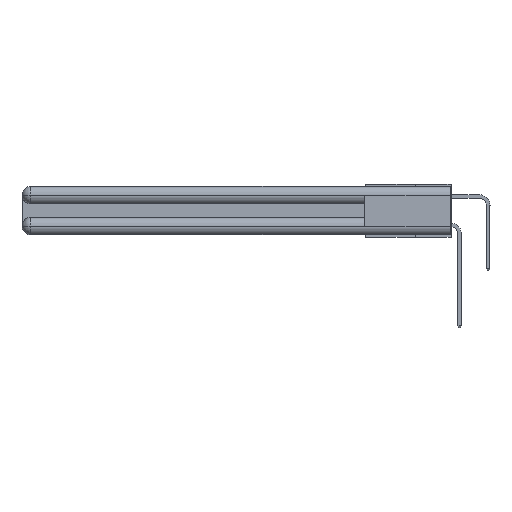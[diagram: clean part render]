
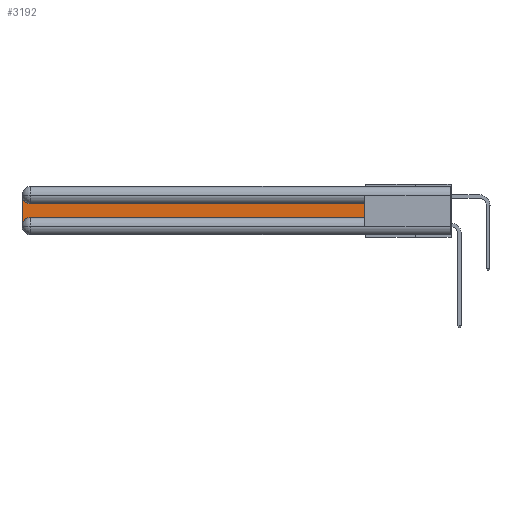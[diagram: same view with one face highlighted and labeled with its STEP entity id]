
A CAD part, left-side view. The second image highlights one B-rep face of the part: STEP entity #3192.
In plain terms, the highlighted planar face has unit normal (-1, 0, 0).
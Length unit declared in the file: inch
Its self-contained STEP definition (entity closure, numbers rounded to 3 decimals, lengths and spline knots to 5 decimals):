
#1713 = VECTOR ( 'NONE', #18691, 39.37008 ) ;
#2190 = CARTESIAN_POINT ( 'NONE',  ( 0.075, 3., -0.2175 ) ) ;
#2395 = EDGE_CURVE ( 'NONE', #20984, #5976, #14051, .T. ) ;
#3192 = ADVANCED_FACE ( 'NONE', ( #27639 ), #4810, .F. ) ;
#3411 = EDGE_CURVE ( 'NONE', #8642, #9436, #4310, .T. ) ;
#3668 = DIRECTION ( 'NONE',  ( 1., 0., 0. ) ) ;
#4007 = ORIENTED_EDGE ( 'NONE', *, *, #29626, .T. ) ;
#4063 = LINE ( 'NONE', #9026, #12921 ) ;
#4310 = LINE ( 'NONE', #8842, #8008 ) ;
#4623 = ORIENTED_EDGE ( 'NONE', *, *, #2395, .T. ) ;
#4810 = PLANE ( 'NONE',  #21521 ) ;
#5691 = VECTOR ( 'NONE', #16833, 39.37008 ) ;
#5976 = VERTEX_POINT ( 'NONE', #21684 ) ;
#6673 = AXIS2_PLACEMENT_3D ( 'NONE', #17833, #3668, #18143 ) ;
#7159 = CARTESIAN_POINT ( 'NONE',  ( 0.075, 3., -0.2775 ) ) ;
#7189 = DIRECTION ( 'NONE',  ( 0., 0., -1. ) ) ;
#8008 = VECTOR ( 'NONE', #10997, 39.37008 ) ;
#8022 = VERTEX_POINT ( 'NONE', #20766 ) ;
#8642 = VERTEX_POINT ( 'NONE', #24124 ) ;
#8842 = CARTESIAN_POINT ( 'NONE',  ( 0.075, 0.6, -0.2175 ) ) ;
#9026 = CARTESIAN_POINT ( 'NONE',  ( 0.075, 0.6, -0.1225 ) ) ;
#9436 = VERTEX_POINT ( 'NONE', #25523 ) ;
#10997 = DIRECTION ( 'NONE',  ( 0., -1., 0. ) ) ;
#12921 = VECTOR ( 'NONE', #20890, 39.37008 ) ;
#14051 = CIRCLE ( 'NONE', #6673, 0.06 ) ;
#16808 = EDGE_LOOP ( 'NONE', ( #28872, #4623, #4007, #26533, #24657, #18396 ) ) ;
#16833 = DIRECTION ( 'NONE',  ( 0., 0., 1. ) ) ;
#17174 = LINE ( 'NONE', #19285, #5691 ) ;
#17833 = CARTESIAN_POINT ( 'NONE',  ( 0.075, 2.94, -0.0625 ) ) ;
#18143 = DIRECTION ( 'NONE',  ( 0., 0., -1. ) ) ;
#18396 = ORIENTED_EDGE ( 'NONE', *, *, #29679, .T. ) ;
#18398 = CIRCLE ( 'NONE', #20300, 0.06 ) ;
#18691 = DIRECTION ( 'NONE',  ( 0., 0., -1. ) ) ;
#19285 = CARTESIAN_POINT ( 'NONE',  ( 0.075, 0.6, -0.2175 ) ) ;
#19967 = CARTESIAN_POINT ( 'NONE',  ( 0.075, 2.94, -0.1225 ) ) ;
#20300 = AXIS2_PLACEMENT_3D ( 'NONE', #29688, #24712, #29596 ) ;
#20766 = CARTESIAN_POINT ( 'NONE',  ( 0.075, 0.6, -0.1225 ) ) ;
#20890 = DIRECTION ( 'NONE',  ( 0., 1., 0. ) ) ;
#20984 = VERTEX_POINT ( 'NONE', #19967 ) ;
#21521 = AXIS2_PLACEMENT_3D ( 'NONE', #23800, #25966, #7189 ) ;
#21684 = CARTESIAN_POINT ( 'NONE',  ( 0.075, 3., -0.0625 ) ) ;
#23083 = LINE ( 'NONE', #2190, #1713 ) ;
#23800 = CARTESIAN_POINT ( 'NONE',  ( 0.075, 3., -0.1225 ) ) ;
#24124 = CARTESIAN_POINT ( 'NONE',  ( 0.075, 2.94, -0.2175 ) ) ;
#24657 = ORIENTED_EDGE ( 'NONE', *, *, #3411, .T. ) ;
#24712 = DIRECTION ( 'NONE',  ( 1., 0., 0. ) ) ;
#25523 = CARTESIAN_POINT ( 'NONE',  ( 0.075, 0.6, -0.2175 ) ) ;
#25966 = DIRECTION ( 'NONE',  ( 1., 0., 0. ) ) ;
#26533 = ORIENTED_EDGE ( 'NONE', *, *, #28309, .T. ) ;
#26898 = EDGE_CURVE ( 'NONE', #8022, #20984, #4063, .T. ) ;
#27639 = FACE_OUTER_BOUND ( 'NONE', #16808, .T. ) ;
#28072 = VERTEX_POINT ( 'NONE', #7159 ) ;
#28309 = EDGE_CURVE ( 'NONE', #28072, #8642, #18398, .T. ) ;
#28872 = ORIENTED_EDGE ( 'NONE', *, *, #26898, .T. ) ;
#29596 = DIRECTION ( 'NONE',  ( 0., 0., -1. ) ) ;
#29626 = EDGE_CURVE ( 'NONE', #5976, #28072, #23083, .T. ) ;
#29679 = EDGE_CURVE ( 'NONE', #9436, #8022, #17174, .T. ) ;
#29688 = CARTESIAN_POINT ( 'NONE',  ( 0.075, 2.94, -0.2775 ) ) ;
